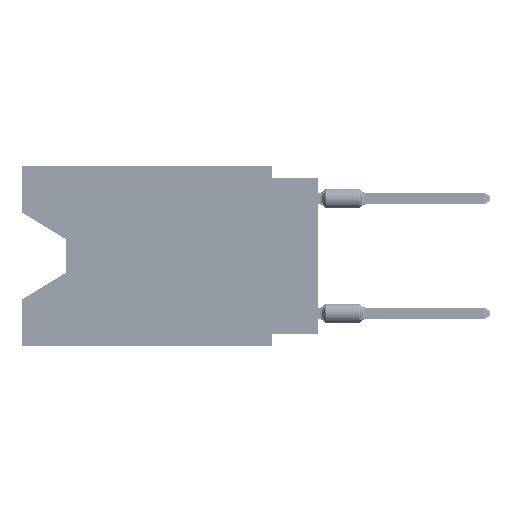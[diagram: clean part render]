
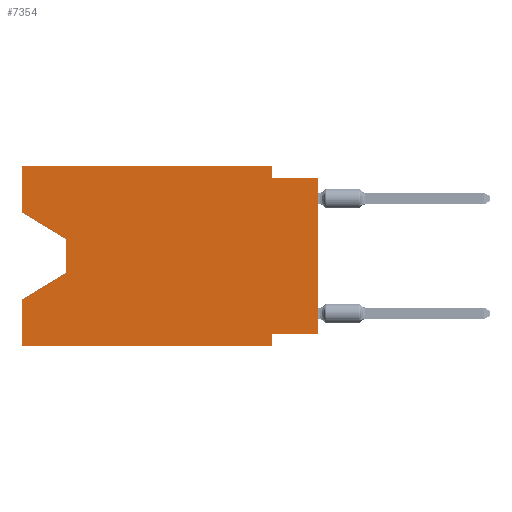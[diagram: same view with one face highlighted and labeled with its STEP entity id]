
A CAD part, left-side view. The second image highlights one B-rep face of the part: STEP entity #7354.
In plain terms, the highlighted planar face has unit normal (-1, 0, 0).
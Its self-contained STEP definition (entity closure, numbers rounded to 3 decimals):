
#634 = CARTESIAN_POINT ( 'NONE',  ( 0., 2.54, -9.906 ) ) ;
#676 = CARTESIAN_POINT ( 'NONE',  ( 0., 2.54, 0. ) ) ;
#815 = DIRECTION ( 'NONE',  ( 0., 0., 1. ) ) ;
#877 = ORIENTED_EDGE ( 'NONE', *, *, #18336, .F. ) ;
#1489 = LINE ( 'NONE', #74118, #44627 ) ;
#1713 = LINE ( 'NONE', #67562, #14467 ) ;
#1742 = VERTEX_POINT ( 'NONE', #676 ) ;
#2701 = CARTESIAN_POINT ( 'NONE',  ( 0., 2.54, -9.271 ) ) ;
#4714 = VECTOR ( 'NONE', #60870, 1000. ) ;
#5836 = VERTEX_POINT ( 'NONE', #10550 ) ;
#6924 = VERTEX_POINT ( 'NONE', #36642 ) ;
#7354 = ADVANCED_FACE ( 'NONE', ( #48121 ), #66893, .F. ) ;
#8504 = CARTESIAN_POINT ( 'NONE',  ( 0., 2.54, -0.635 ) ) ;
#8988 = LINE ( 'NONE', #45678, #72459 ) ;
#9154 = VECTOR ( 'NONE', #19274, 1000. ) ;
#9895 = DIRECTION ( 'NONE',  ( 0., 0., -1. ) ) ;
#10550 = CARTESIAN_POINT ( 'NONE',  ( 0., 16.383, -9.906 ) ) ;
#11044 = CARTESIAN_POINT ( 'NONE',  ( 0., 16.383, 0. ) ) ;
#12221 = DIRECTION ( 'NONE',  ( 0., -1., 0. ) ) ;
#13204 = VERTEX_POINT ( 'NONE', #73463 ) ;
#13565 = CARTESIAN_POINT ( 'NONE',  ( 0., 13.97, -4.013 ) ) ;
#14467 = VECTOR ( 'NONE', #50378, 1000. ) ;
#14750 = CARTESIAN_POINT ( 'NONE',  ( 0., 0., 0. ) ) ;
#15982 = ORIENTED_EDGE ( 'NONE', *, *, #71224, .T. ) ;
#16515 = CARTESIAN_POINT ( 'NONE',  ( 0., 2.54, -9.906 ) ) ;
#18336 = EDGE_CURVE ( 'NONE', #1742, #51304, #1489, .T. ) ;
#19274 = DIRECTION ( 'NONE',  ( 0., 0., 1. ) ) ;
#20395 = VERTEX_POINT ( 'NONE', #73542 ) ;
#21462 = VERTEX_POINT ( 'NONE', #16515 ) ;
#23020 = LINE ( 'NONE', #11044, #40019 ) ;
#23795 = CARTESIAN_POINT ( 'NONE',  ( 0., 16.383, 0. ) ) ;
#25353 = LINE ( 'NONE', #634, #4714 ) ;
#26751 = VECTOR ( 'NONE', #815, 1000. ) ;
#26799 = EDGE_CURVE ( 'NONE', #6924, #20395, #43497, .T. ) ;
#27397 = CARTESIAN_POINT ( 'NONE',  ( 0., 16.383, 0. ) ) ;
#28358 = LINE ( 'NONE', #41084, #35013 ) ;
#29148 = ORIENTED_EDGE ( 'NONE', *, *, #68150, .F. ) ;
#30699 = VERTEX_POINT ( 'NONE', #27397 ) ;
#31898 = LINE ( 'NONE', #14750, #26751 ) ;
#32887 = EDGE_CURVE ( 'NONE', #72175, #69706, #31898, .T. ) ;
#33625 = ORIENTED_EDGE ( 'NONE', *, *, #40694, .T. ) ;
#35013 = VECTOR ( 'NONE', #45901, 1000. ) ;
#36177 = AXIS2_PLACEMENT_3D ( 'NONE', #23795, #41744, #66491 ) ;
#36642 = CARTESIAN_POINT ( 'NONE',  ( 0., 13.97, -5.893 ) ) ;
#39105 = CARTESIAN_POINT ( 'NONE',  ( 0., 13.97, -5.893 ) ) ;
#39268 = CARTESIAN_POINT ( 'NONE',  ( 0., 16.383, -2.546 ) ) ;
#40019 = VECTOR ( 'NONE', #12221, 1000. ) ;
#40206 = CARTESIAN_POINT ( 'NONE',  ( 0., 13.97, -4.013 ) ) ;
#40694 = EDGE_CURVE ( 'NONE', #5836, #21462, #59280, .T. ) ;
#40934 = CARTESIAN_POINT ( 'NONE',  ( 0., 0., -9.271 ) ) ;
#41084 = CARTESIAN_POINT ( 'NONE',  ( 0., 0., -0.635 ) ) ;
#41382 = VECTOR ( 'NONE', #45070, 1000. ) ;
#41717 = VECTOR ( 'NONE', #62061, 1000. ) ;
#41744 = DIRECTION ( 'NONE',  ( 1., 0., 0. ) ) ;
#43497 = LINE ( 'NONE', #39105, #41382 ) ;
#44627 = VECTOR ( 'NONE', #50551, 1000. ) ;
#44702 = ORIENTED_EDGE ( 'NONE', *, *, #47278, .F. ) ;
#45070 = DIRECTION ( 'NONE',  ( 0., 0.855, -0.519 ) ) ;
#45678 = CARTESIAN_POINT ( 'NONE',  ( 0., 0., -9.271 ) ) ;
#45901 = DIRECTION ( 'NONE',  ( 0., -1., 0. ) ) ;
#47278 = EDGE_CURVE ( 'NONE', #72175, #50467, #8988, .T. ) ;
#48121 = FACE_OUTER_BOUND ( 'NONE', #67442, .T. ) ;
#49999 = LINE ( 'NONE', #55608, #9154 ) ;
#50378 = DIRECTION ( 'NONE',  ( 0., 0., 1. ) ) ;
#50467 = VERTEX_POINT ( 'NONE', #2701 ) ;
#50551 = DIRECTION ( 'NONE',  ( 0., 0., -1. ) ) ;
#51304 = VERTEX_POINT ( 'NONE', #8504 ) ;
#55460 = VECTOR ( 'NONE', #9895, 1000. ) ;
#55608 = CARTESIAN_POINT ( 'NONE',  ( 0., 16.383, 0. ) ) ;
#57773 = LINE ( 'NONE', #40206, #55460 ) ;
#59280 = LINE ( 'NONE', #72432, #73063 ) ;
#60870 = DIRECTION ( 'NONE',  ( 0., 0., -1. ) ) ;
#61176 = EDGE_CURVE ( 'NONE', #5836, #20395, #49999, .T. ) ;
#61930 = ORIENTED_EDGE ( 'NONE', *, *, #63770, .F. ) ;
#62061 = DIRECTION ( 'NONE',  ( 0., -0.855, -0.519 ) ) ;
#62393 = ORIENTED_EDGE ( 'NONE', *, *, #32887, .T. ) ;
#62921 = ORIENTED_EDGE ( 'NONE', *, *, #26799, .T. ) ;
#63770 = EDGE_CURVE ( 'NONE', #30699, #1742, #23020, .T. ) ;
#64055 = DIRECTION ( 'NONE',  ( 0., 1., 0. ) ) ;
#64964 = EDGE_CURVE ( 'NONE', #71527, #6924, #57773, .T. ) ;
#66491 = DIRECTION ( 'NONE',  ( 0., 0., -1. ) ) ;
#66838 = DIRECTION ( 'NONE',  ( 0., -1., 0. ) ) ;
#66893 = PLANE ( 'NONE',  #36177 ) ;
#67442 = EDGE_LOOP ( 'NONE', ( #15982, #75471, #62921, #76957, #33625, #70924, #44702, #62393, #29148, #877, #61930, #70154 ) ) ;
#67562 = CARTESIAN_POINT ( 'NONE',  ( 0., 16.383, 0. ) ) ;
#68150 = EDGE_CURVE ( 'NONE', #51304, #69706, #28358, .T. ) ;
#69617 = LINE ( 'NONE', #39268, #41717 ) ;
#69706 = VERTEX_POINT ( 'NONE', #72711 ) ;
#70154 = ORIENTED_EDGE ( 'NONE', *, *, #78404, .F. ) ;
#70924 = ORIENTED_EDGE ( 'NONE', *, *, #72242, .F. ) ;
#71224 = EDGE_CURVE ( 'NONE', #13204, #71527, #69617, .T. ) ;
#71527 = VERTEX_POINT ( 'NONE', #13565 ) ;
#72175 = VERTEX_POINT ( 'NONE', #40934 ) ;
#72242 = EDGE_CURVE ( 'NONE', #50467, #21462, #25353, .T. ) ;
#72432 = CARTESIAN_POINT ( 'NONE',  ( 0., 16.383, -9.906 ) ) ;
#72459 = VECTOR ( 'NONE', #64055, 1000. ) ;
#72711 = CARTESIAN_POINT ( 'NONE',  ( 0., 0., -0.635 ) ) ;
#73063 = VECTOR ( 'NONE', #66838, 1000. ) ;
#73463 = CARTESIAN_POINT ( 'NONE',  ( 0., 16.383, -2.546 ) ) ;
#73542 = CARTESIAN_POINT ( 'NONE',  ( 0., 16.383, -7.36 ) ) ;
#74118 = CARTESIAN_POINT ( 'NONE',  ( 0., 2.54, 0. ) ) ;
#75471 = ORIENTED_EDGE ( 'NONE', *, *, #64964, .T. ) ;
#76957 = ORIENTED_EDGE ( 'NONE', *, *, #61176, .F. ) ;
#78404 = EDGE_CURVE ( 'NONE', #13204, #30699, #1713, .T. ) ;
